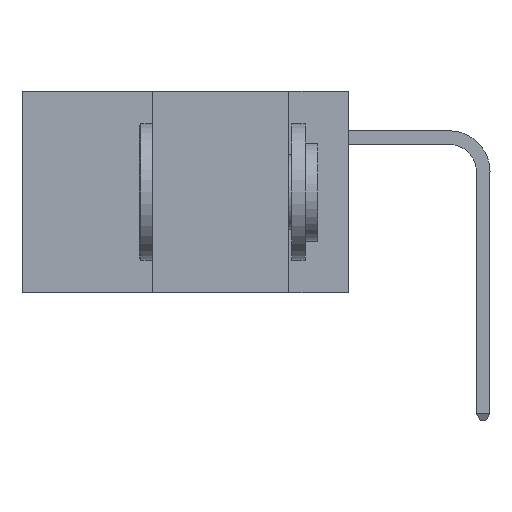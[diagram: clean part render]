
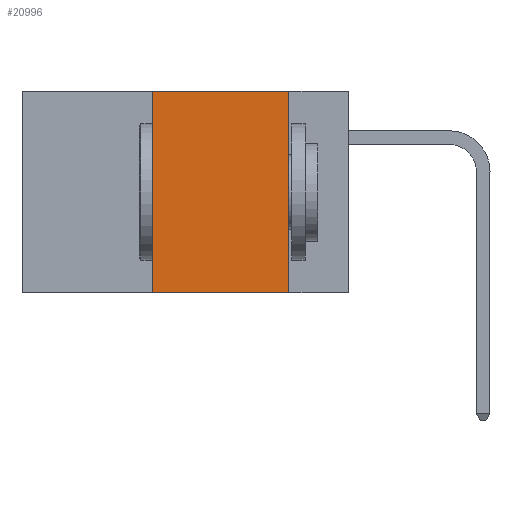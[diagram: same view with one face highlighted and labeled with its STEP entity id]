
A CAD part, left-side view. The second image highlights one B-rep face of the part: STEP entity #20996.
In plain terms, the highlighted planar face has unit normal (-1, 0, 0).
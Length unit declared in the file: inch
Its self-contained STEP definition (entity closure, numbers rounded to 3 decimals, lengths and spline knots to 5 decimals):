
#26 = CARTESIAN_POINT ( 'NONE',  ( 0., 0.36, -0.37 ) ) ;
#166 = LINE ( 'NONE', #2497, #17792 ) ;
#420 = EDGE_CURVE ( 'NONE', #16616, #10860, #20161, .T. ) ;
#1162 = EDGE_CURVE ( 'NONE', #1282, #10860, #166, .T. ) ;
#1282 = VERTEX_POINT ( 'NONE', #26 ) ;
#1584 = DIRECTION ( 'NONE',  ( 0., 0., 1. ) ) ;
#1960 = CARTESIAN_POINT ( 'NONE',  ( 0., 0.11, -0.37 ) ) ;
#2226 = DIRECTION ( 'NONE',  ( 0., -1., 0. ) ) ;
#2497 = CARTESIAN_POINT ( 'NONE',  ( 0., 0.6, -0.37 ) ) ;
#2729 = EDGE_LOOP ( 'NONE', ( #14589, #15103, #6750, #7281 ) ) ;
#6032 = VECTOR ( 'NONE', #10519, 39.37008 ) ;
#6541 = LINE ( 'NONE', #8821, #6032 ) ;
#6750 = ORIENTED_EDGE ( 'NONE', *, *, #12026, .F. ) ;
#6874 = VECTOR ( 'NONE', #21891, 39.37008 ) ;
#7281 = ORIENTED_EDGE ( 'NONE', *, *, #1162, .T. ) ;
#7933 = DIRECTION ( 'NONE',  ( 0., 0., -1. ) ) ;
#8821 = CARTESIAN_POINT ( 'NONE',  ( 0., 0.6, 0. ) ) ;
#9175 = CARTESIAN_POINT ( 'NONE',  ( 0., 0.36, 0. ) ) ;
#9425 = AXIS2_PLACEMENT_3D ( 'NONE', #12934, #17909, #7933 ) ;
#10519 = DIRECTION ( 'NONE',  ( 0., -1., 0. ) ) ;
#10860 = VERTEX_POINT ( 'NONE', #1960 ) ;
#10959 = VERTEX_POINT ( 'NONE', #9175 ) ;
#11286 = FACE_OUTER_BOUND ( 'NONE', #2729, .T. ) ;
#12026 = EDGE_CURVE ( 'NONE', #1282, #10959, #16470, .T. ) ;
#12063 = VECTOR ( 'NONE', #1584, 39.37008 ) ;
#12117 = EDGE_CURVE ( 'NONE', #10959, #16616, #6541, .T. ) ;
#12934 = CARTESIAN_POINT ( 'NONE',  ( 0., 0.6, 0. ) ) ;
#14589 = ORIENTED_EDGE ( 'NONE', *, *, #420, .F. ) ;
#15103 = ORIENTED_EDGE ( 'NONE', *, *, #12117, .F. ) ;
#16252 = PLANE ( 'NONE',  #9425 ) ;
#16470 = LINE ( 'NONE', #21889, #12063 ) ;
#16616 = VERTEX_POINT ( 'NONE', #20777 ) ;
#17792 = VECTOR ( 'NONE', #2226, 39.37008 ) ;
#17909 = DIRECTION ( 'NONE',  ( 1., 0., 0. ) ) ;
#20161 = LINE ( 'NONE', #21845, #6874 ) ;
#20777 = CARTESIAN_POINT ( 'NONE',  ( 0., 0.11, 0. ) ) ;
#20996 = ADVANCED_FACE ( 'NONE', ( #11286 ), #16252, .F. ) ;
#21845 = CARTESIAN_POINT ( 'NONE',  ( 0., 0.11, 0. ) ) ;
#21889 = CARTESIAN_POINT ( 'NONE',  ( 0., 0.36, 0. ) ) ;
#21891 = DIRECTION ( 'NONE',  ( 0., 0., -1. ) ) ;
